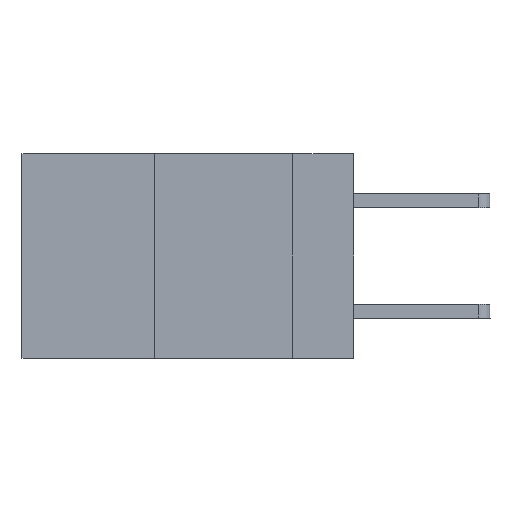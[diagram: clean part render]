
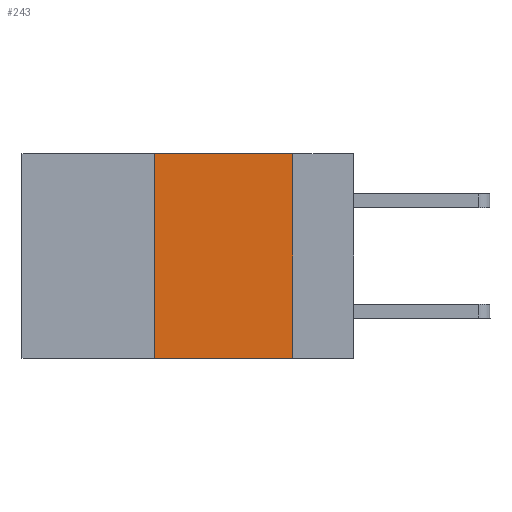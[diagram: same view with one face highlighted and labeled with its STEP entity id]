
A CAD part, left-side view. The second image highlights one B-rep face of the part: STEP entity #243.
In plain terms, the highlighted planar face has unit normal (-1, 0, 0).
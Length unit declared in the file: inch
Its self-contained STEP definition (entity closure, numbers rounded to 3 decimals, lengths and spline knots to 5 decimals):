
#243 = ADVANCED_FACE ( 'NONE', ( #2070 ), #2447, .F. ) ;
#331 = CARTESIAN_POINT ( 'NONE',  ( 0., 0.36, 0. ) ) ;
#563 = ORIENTED_EDGE ( 'NONE', *, *, #9181, .F. ) ;
#1521 = CARTESIAN_POINT ( 'NONE',  ( 0., 0.6, 0. ) ) ;
#1615 = VECTOR ( 'NONE', #10131, 39.37008 ) ;
#2070 = FACE_OUTER_BOUND ( 'NONE', #6730, .T. ) ;
#2201 = DIRECTION ( 'NONE',  ( 0., 0., -1. ) ) ;
#2447 = PLANE ( 'NONE',  #6625 ) ;
#2591 = DIRECTION ( 'NONE',  ( 1., 0., 0. ) ) ;
#2990 = LINE ( 'NONE', #1521, #1615 ) ;
#3336 = VERTEX_POINT ( 'NONE', #7112 ) ;
#3344 = CARTESIAN_POINT ( 'NONE',  ( 0., 0.6, 0. ) ) ;
#3422 = DIRECTION ( 'NONE',  ( 0., -1., 0. ) ) ;
#3756 = EDGE_CURVE ( 'NONE', #10105, #5425, #6526, .T. ) ;
#3842 = DIRECTION ( 'NONE',  ( 0., 0., 1. ) ) ;
#5039 = CARTESIAN_POINT ( 'NONE',  ( 0., 0.36, -0.37 ) ) ;
#5425 = VERTEX_POINT ( 'NONE', #331 ) ;
#5430 = ORIENTED_EDGE ( 'NONE', *, *, #6727, .T. ) ;
#6090 = LINE ( 'NONE', #8606, #8425 ) ;
#6165 = ORIENTED_EDGE ( 'NONE', *, *, #6430, .F. ) ;
#6430 = EDGE_CURVE ( 'NONE', #8965, #3336, #6090, .T. ) ;
#6526 = LINE ( 'NONE', #6948, #7280 ) ;
#6625 = AXIS2_PLACEMENT_3D ( 'NONE', #3344, #2591, #7134 ) ;
#6727 = EDGE_CURVE ( 'NONE', #10105, #3336, #7439, .T. ) ;
#6730 = EDGE_LOOP ( 'NONE', ( #6165, #563, #8483, #5430 ) ) ;
#6948 = CARTESIAN_POINT ( 'NONE',  ( 0., 0.36, 0. ) ) ;
#7112 = CARTESIAN_POINT ( 'NONE',  ( 0., 0.11, -0.37 ) ) ;
#7134 = DIRECTION ( 'NONE',  ( 0., 0., -1. ) ) ;
#7280 = VECTOR ( 'NONE', #3842, 39.37008 ) ;
#7439 = LINE ( 'NONE', #8043, #8533 ) ;
#8043 = CARTESIAN_POINT ( 'NONE',  ( 0., 0.6, -0.37 ) ) ;
#8425 = VECTOR ( 'NONE', #2201, 39.37008 ) ;
#8483 = ORIENTED_EDGE ( 'NONE', *, *, #3756, .F. ) ;
#8533 = VECTOR ( 'NONE', #3422, 39.37008 ) ;
#8606 = CARTESIAN_POINT ( 'NONE',  ( 0., 0.11, 0. ) ) ;
#8965 = VERTEX_POINT ( 'NONE', #9027 ) ;
#9027 = CARTESIAN_POINT ( 'NONE',  ( 0., 0.11, 0. ) ) ;
#9181 = EDGE_CURVE ( 'NONE', #5425, #8965, #2990, .T. ) ;
#10105 = VERTEX_POINT ( 'NONE', #5039 ) ;
#10131 = DIRECTION ( 'NONE',  ( 0., -1., 0. ) ) ;
